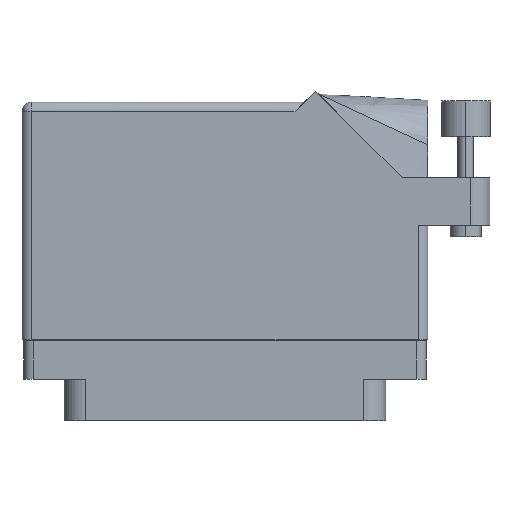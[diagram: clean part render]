
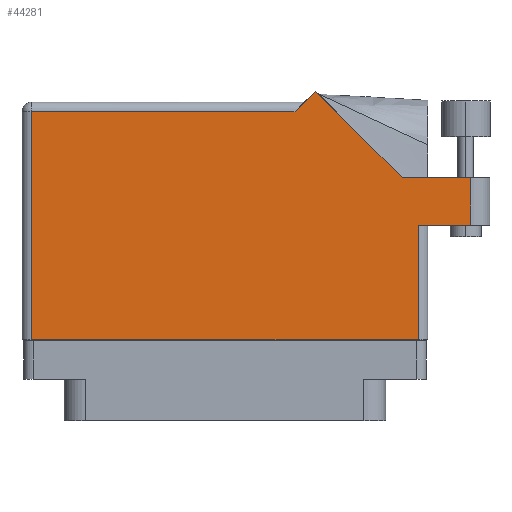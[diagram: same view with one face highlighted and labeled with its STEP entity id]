
A CAD part, front view. The second image highlights one B-rep face of the part: STEP entity #44281.
In plain terms, the highlighted face is planar.
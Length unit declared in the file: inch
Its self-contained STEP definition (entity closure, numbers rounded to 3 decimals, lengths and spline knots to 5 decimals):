
#547 = CARTESIAN_POINT ( 'NONE',  ( -1.244, -0.1, 0.455 ) ) ;
#666 = VECTOR ( 'NONE', #23083, 39.37008 ) ;
#717 = EDGE_CURVE ( 'NONE', #27435, #45995, #46474, .T. ) ;
#1597 = VERTEX_POINT ( 'NONE', #34866 ) ;
#1790 = ORIENTED_EDGE ( 'NONE', *, *, #42609, .T. ) ;
#2167 = CARTESIAN_POINT ( 'NONE',  ( 0.513, 1.43, 0.455 ) ) ;
#2406 = VECTOR ( 'NONE', #31661, 39.37008 ) ;
#4635 = VERTEX_POINT ( 'NONE', #13815 ) ;
#4761 = VECTOR ( 'NONE', #46169, 39.37008 ) ;
#5640 = CARTESIAN_POINT ( 'NONE',  ( -1.244, 1.368, 0.455 ) ) ;
#5714 = ORIENTED_EDGE ( 'NONE', *, *, #12187, .T. ) ;
#6142 = EDGE_CURVE ( 'NONE', #10551, #1597, #16834, .T. ) ;
#6641 = VECTOR ( 'NONE', #39685, 39.37008 ) ;
#8198 = LINE ( 'NONE', #40964, #666 ) ;
#9818 = AXIS2_PLACEMENT_3D ( 'NONE', #36492, #43956, #36163 ) ;
#10004 = EDGE_CURVE ( 'NONE', #30312, #47485, #8198, .T. ) ;
#10273 = PLANE ( 'NONE',  #9818 ) ;
#10551 = VERTEX_POINT ( 'NONE', #27713 ) ;
#10679 = LINE ( 'NONE', #36036, #6641 ) ;
#10683 = DIRECTION ( 'NONE',  ( -0.707, 0.707, 0. ) ) ;
#10999 = CARTESIAN_POINT ( 'NONE',  ( 1.14042, 0.944, 0.455 ) ) ;
#12004 = DIRECTION ( 'NONE',  ( 0., -1., 0. ) ) ;
#12187 = EDGE_CURVE ( 'NONE', #4635, #30312, #16298, .T. ) ;
#13474 = ORIENTED_EDGE ( 'NONE', *, *, #24677, .T. ) ;
#13815 = CARTESIAN_POINT ( 'NONE',  ( 1.581, 0.637, 0.455 ) ) ;
#14218 = DIRECTION ( 'NONE',  ( 0., 1., 0. ) ) ;
#14320 = ORIENTED_EDGE ( 'NONE', *, *, #36867, .T. ) ;
#14826 = EDGE_CURVE ( 'NONE', #47485, #10551, #21107, .T. ) ;
#16286 = CARTESIAN_POINT ( 'NONE',  ( 1.244, 0.637, 0.455 ) ) ;
#16289 = CARTESIAN_POINT ( 'NONE',  ( 1.14042, 0.944, 0.455 ) ) ;
#16298 = LINE ( 'NONE', #44363, #22114 ) ;
#16834 = LINE ( 'NONE', #2167, #2406 ) ;
#20770 = CARTESIAN_POINT ( 'NONE',  ( -1.306, 1.368, 0.455 ) ) ;
#21107 = LINE ( 'NONE', #10999, #36817 ) ;
#22114 = VECTOR ( 'NONE', #14218, 39.37008 ) ;
#22764 = VERTEX_POINT ( 'NONE', #5640 ) ;
#23083 = DIRECTION ( 'NONE',  ( -1., 0., 0. ) ) ;
#23147 = FACE_OUTER_BOUND ( 'NONE', #30540, .T. ) ;
#23169 = VECTOR ( 'NONE', #41803, 39.37008 ) ;
#24677 = EDGE_CURVE ( 'NONE', #1597, #22764, #26117, .T. ) ;
#26058 = LINE ( 'NONE', #35003, #23169 ) ;
#26117 = LINE ( 'NONE', #20770, #4761 ) ;
#26867 = CARTESIAN_POINT ( 'NONE',  ( -1.244, -0.1, 0.455 ) ) ;
#27013 = CARTESIAN_POINT ( 'NONE',  ( 1.244, -0.1, 0.455 ) ) ;
#27058 = ORIENTED_EDGE ( 'NONE', *, *, #43296, .T. ) ;
#27435 = VERTEX_POINT ( 'NONE', #27013 ) ;
#27713 = CARTESIAN_POINT ( 'NONE',  ( 0.58371, 1.50071, 0.455 ) ) ;
#28874 = ORIENTED_EDGE ( 'NONE', *, *, #10004, .T. ) ;
#29073 = ORIENTED_EDGE ( 'NONE', *, *, #717, .T. ) ;
#29129 = CARTESIAN_POINT ( 'NONE',  ( 1.581, 0.944, 0.455 ) ) ;
#30134 = VECTOR ( 'NONE', #12004, 39.37008 ) ;
#30312 = VERTEX_POINT ( 'NONE', #29129 ) ;
#30423 = ORIENTED_EDGE ( 'NONE', *, *, #14826, .T. ) ;
#30540 = EDGE_LOOP ( 'NONE', ( #14320, #5714, #28874, #30423, #31109, #13474, #27058, #1790, #29073 ) ) ;
#30866 = CARTESIAN_POINT ( 'NONE',  ( 1.244, 0.637, 0.455 ) ) ;
#31109 = ORIENTED_EDGE ( 'NONE', *, *, #6142, .T. ) ;
#31661 = DIRECTION ( 'NONE',  ( -0.707, -0.707, 0. ) ) ;
#34866 = CARTESIAN_POINT ( 'NONE',  ( 0.451, 1.368, 0.455 ) ) ;
#35003 = CARTESIAN_POINT ( 'NONE',  ( -1.306, -0.1, 0.455 ) ) ;
#36036 = CARTESIAN_POINT ( 'NONE',  ( 1.306, 0.637, 0.455 ) ) ;
#36163 = DIRECTION ( 'NONE',  ( -1., 0., 0. ) ) ;
#36492 = CARTESIAN_POINT ( 'NONE',  ( -1.306, 1.43, 0.455 ) ) ;
#36817 = VECTOR ( 'NONE', #10683, 39.37008 ) ;
#36867 = EDGE_CURVE ( 'NONE', #45995, #4635, #10679, .T. ) ;
#37554 = VERTEX_POINT ( 'NONE', #26867 ) ;
#38696 = LINE ( 'NONE', #547, #30134 ) ;
#39685 = DIRECTION ( 'NONE',  ( 1., 0., 0. ) ) ;
#40964 = CARTESIAN_POINT ( 'NONE',  ( 1.706, 0.944, 0.455 ) ) ;
#41803 = DIRECTION ( 'NONE',  ( 1., 0., 0. ) ) ;
#42405 = DIRECTION ( 'NONE',  ( 0., 1., 0. ) ) ;
#42609 = EDGE_CURVE ( 'NONE', #37554, #27435, #26058, .T. ) ;
#43296 = EDGE_CURVE ( 'NONE', #22764, #37554, #38696, .T. ) ;
#43956 = DIRECTION ( 'NONE',  ( 0., 0., -1. ) ) ;
#44281 = ADVANCED_FACE ( 'NONE', ( #23147 ), #10273, .F. ) ;
#44363 = CARTESIAN_POINT ( 'NONE',  ( 1.581, 0.944, 0.455 ) ) ;
#45995 = VERTEX_POINT ( 'NONE', #30866 ) ;
#46169 = DIRECTION ( 'NONE',  ( -1., 0., 0. ) ) ;
#46474 = LINE ( 'NONE', #16286, #47027 ) ;
#47027 = VECTOR ( 'NONE', #42405, 39.37008 ) ;
#47485 = VERTEX_POINT ( 'NONE', #16289 ) ;
